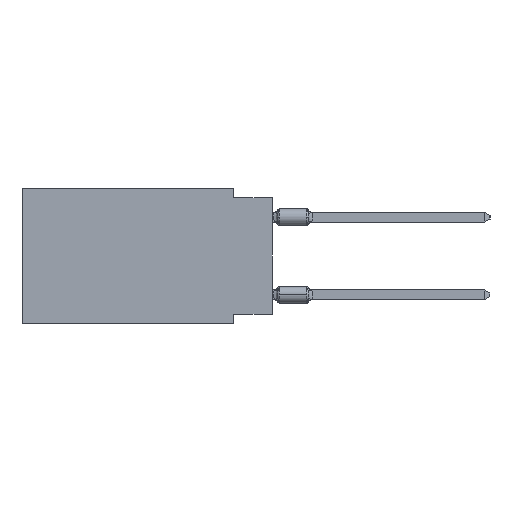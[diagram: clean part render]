
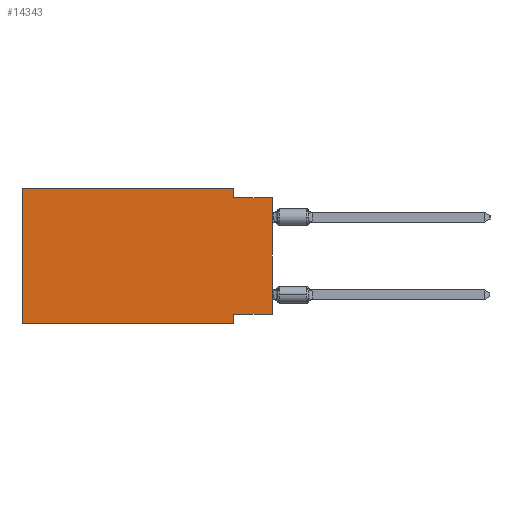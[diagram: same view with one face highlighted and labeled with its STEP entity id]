
A CAD part, left-side view. The second image highlights one B-rep face of the part: STEP entity #14343.
In plain terms, the highlighted planar face has unit normal (-1, 0, 0).
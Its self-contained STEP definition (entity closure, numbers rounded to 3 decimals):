
#583 = VERTEX_POINT ( 'NONE', #17264 ) ;
#1215 = CARTESIAN_POINT ( 'NONE',  ( 0., 2.54, -8.89 ) ) ;
#3032 = CARTESIAN_POINT ( 'NONE',  ( 0., 2.54, -0.635 ) ) ;
#3938 = VERTEX_POINT ( 'NONE', #22507 ) ;
#4388 = AXIS2_PLACEMENT_3D ( 'NONE', #11349, #6331, #14164 ) ;
#4446 = FACE_OUTER_BOUND ( 'NONE', #29381, .T. ) ;
#4546 = DIRECTION ( 'NONE',  ( 0., 0., -1. ) ) ;
#5367 = DIRECTION ( 'NONE',  ( 0., -1., 0. ) ) ;
#5745 = LINE ( 'NONE', #25179, #17820 ) ;
#6331 = DIRECTION ( 'NONE',  ( 1., 0., 0. ) ) ;
#6386 = LINE ( 'NONE', #6550, #25529 ) ;
#6486 = EDGE_CURVE ( 'NONE', #12414, #16699, #8149, .T. ) ;
#6550 = CARTESIAN_POINT ( 'NONE',  ( 0., 0., -0.635 ) ) ;
#6719 = EDGE_CURVE ( 'NONE', #8549, #11193, #11195, .T. ) ;
#6727 = ORIENTED_EDGE ( 'NONE', *, *, #6719, .F. ) ;
#7056 = VERTEX_POINT ( 'NONE', #11164 ) ;
#8149 = LINE ( 'NONE', #20656, #22013 ) ;
#8549 = VERTEX_POINT ( 'NONE', #29480 ) ;
#8551 = VECTOR ( 'NONE', #5367, 1000. ) ;
#9919 = VECTOR ( 'NONE', #4546, 1000. ) ;
#10121 = CARTESIAN_POINT ( 'NONE',  ( 0., 0., -8.255 ) ) ;
#10261 = VECTOR ( 'NONE', #16549, 1000. ) ;
#11164 = CARTESIAN_POINT ( 'NONE',  ( 0., 16.383, 0. ) ) ;
#11193 = VERTEX_POINT ( 'NONE', #3032 ) ;
#11195 = LINE ( 'NONE', #18246, #20039 ) ;
#11349 = CARTESIAN_POINT ( 'NONE',  ( 0., 16.383, 0. ) ) ;
#12237 = EDGE_CURVE ( 'NONE', #12414, #583, #16694, .T. ) ;
#12400 = ORIENTED_EDGE ( 'NONE', *, *, #19123, .F. ) ;
#12414 = VERTEX_POINT ( 'NONE', #10121 ) ;
#12735 = LINE ( 'NONE', #16812, #8551 ) ;
#13126 = DIRECTION ( 'NONE',  ( 0., -1., 0. ) ) ;
#14164 = DIRECTION ( 'NONE',  ( 0., 0., -1. ) ) ;
#14343 = ADVANCED_FACE ( 'NONE', ( #4446 ), #16518, .F. ) ;
#14667 = CARTESIAN_POINT ( 'NONE',  ( 0., 16.383, 0. ) ) ;
#15957 = DIRECTION ( 'NONE',  ( 0., -1., 0. ) ) ;
#16312 = VECTOR ( 'NONE', #23930, 1000. ) ;
#16333 = VERTEX_POINT ( 'NONE', #1215 ) ;
#16518 = PLANE ( 'NONE',  #4388 ) ;
#16549 = DIRECTION ( 'NONE',  ( 0., 1., 0. ) ) ;
#16694 = LINE ( 'NONE', #28755, #10261 ) ;
#16699 = VERTEX_POINT ( 'NONE', #28085 ) ;
#16812 = CARTESIAN_POINT ( 'NONE',  ( 0., 16.383, -8.89 ) ) ;
#17232 = EDGE_CURVE ( 'NONE', #11193, #16699, #6386, .T. ) ;
#17264 = CARTESIAN_POINT ( 'NONE',  ( 0., 2.54, -8.255 ) ) ;
#17820 = VECTOR ( 'NONE', #13126, 1000. ) ;
#17833 = DIRECTION ( 'NONE',  ( 0., 0., 1. ) ) ;
#18246 = CARTESIAN_POINT ( 'NONE',  ( 0., 2.54, 0. ) ) ;
#19123 = EDGE_CURVE ( 'NONE', #3938, #7056, #23778, .T. ) ;
#19530 = ORIENTED_EDGE ( 'NONE', *, *, #22982, .F. ) ;
#20039 = VECTOR ( 'NONE', #23115, 1000. ) ;
#20656 = CARTESIAN_POINT ( 'NONE',  ( 0., 0., 0. ) ) ;
#20681 = ORIENTED_EDGE ( 'NONE', *, *, #12237, .F. ) ;
#21003 = LINE ( 'NONE', #26173, #9919 ) ;
#21416 = EDGE_CURVE ( 'NONE', #583, #16333, #21003, .T. ) ;
#21556 = ORIENTED_EDGE ( 'NONE', *, *, #21416, .F. ) ;
#22013 = VECTOR ( 'NONE', #17833, 1000. ) ;
#22507 = CARTESIAN_POINT ( 'NONE',  ( 0., 16.383, -8.89 ) ) ;
#22982 = EDGE_CURVE ( 'NONE', #7056, #8549, #5745, .T. ) ;
#23115 = DIRECTION ( 'NONE',  ( 0., 0., -1. ) ) ;
#23778 = LINE ( 'NONE', #14667, #16312 ) ;
#23930 = DIRECTION ( 'NONE',  ( 0., 0., 1. ) ) ;
#24934 = EDGE_CURVE ( 'NONE', #3938, #16333, #12735, .T. ) ;
#25179 = CARTESIAN_POINT ( 'NONE',  ( 0., 16.383, 0. ) ) ;
#25529 = VECTOR ( 'NONE', #15957, 1000. ) ;
#26173 = CARTESIAN_POINT ( 'NONE',  ( 0., 2.54, -8.89 ) ) ;
#26370 = ORIENTED_EDGE ( 'NONE', *, *, #24934, .T. ) ;
#28037 = ORIENTED_EDGE ( 'NONE', *, *, #6486, .T. ) ;
#28085 = CARTESIAN_POINT ( 'NONE',  ( 0., 0., -0.635 ) ) ;
#28755 = CARTESIAN_POINT ( 'NONE',  ( 0., 0., -8.255 ) ) ;
#29381 = EDGE_LOOP ( 'NONE', ( #28037, #30939, #6727, #19530, #12400, #26370, #21556, #20681 ) ) ;
#29480 = CARTESIAN_POINT ( 'NONE',  ( 0., 2.54, 0. ) ) ;
#30939 = ORIENTED_EDGE ( 'NONE', *, *, #17232, .F. ) ;
